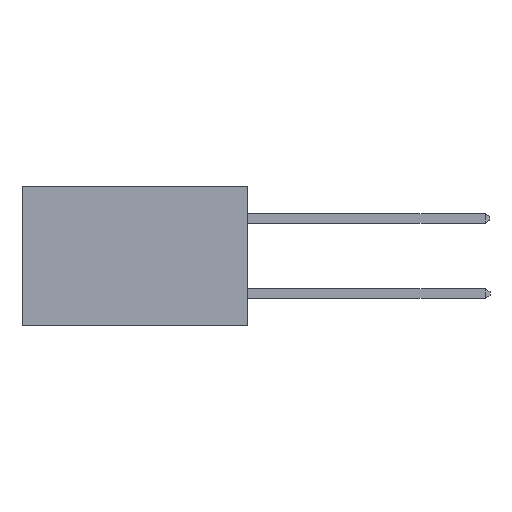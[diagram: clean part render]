
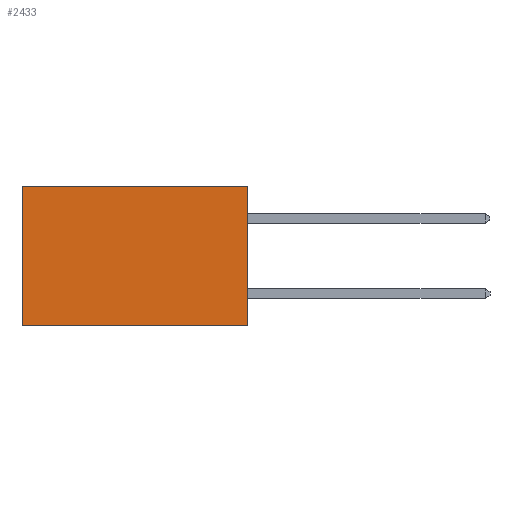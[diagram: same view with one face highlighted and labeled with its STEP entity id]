
A CAD part, left-side view. The second image highlights one B-rep face of the part: STEP entity #2433.
In plain terms, the highlighted planar face has unit normal (-1, 0, 0).
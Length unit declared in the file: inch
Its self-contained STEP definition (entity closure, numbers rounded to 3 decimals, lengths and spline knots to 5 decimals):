
#88 = VECTOR ( 'NONE', #7868, 39.37008 ) ;
#504 = LINE ( 'NONE', #7712, #5541 ) ;
#570 = CARTESIAN_POINT ( 'NONE',  ( 0.2615, 0., 0. ) ) ;
#1166 = CARTESIAN_POINT ( 'NONE',  ( 0.2615, 0.6, -0.37 ) ) ;
#1446 = VECTOR ( 'NONE', #7202, 39.37008 ) ;
#1476 = FACE_OUTER_BOUND ( 'NONE', #3121, .T. ) ;
#1584 = EDGE_CURVE ( 'NONE', #1748, #5989, #6797, .T. ) ;
#1657 = CARTESIAN_POINT ( 'NONE',  ( 0.2615, 0.6, 0. ) ) ;
#1748 = VERTEX_POINT ( 'NONE', #3510 ) ;
#2280 = EDGE_CURVE ( 'NONE', #2652, #6711, #2873, .T. ) ;
#2433 = ADVANCED_FACE ( 'NONE', ( #1476 ), #2938, .F. ) ;
#2652 = VERTEX_POINT ( 'NONE', #570 ) ;
#2756 = AXIS2_PLACEMENT_3D ( 'NONE', #3023, #2908, #2900 ) ;
#2873 = LINE ( 'NONE', #4384, #6101 ) ;
#2900 = DIRECTION ( 'NONE',  ( 0., 0., -1. ) ) ;
#2908 = DIRECTION ( 'NONE',  ( 1., 0., 0. ) ) ;
#2938 = PLANE ( 'NONE',  #2756 ) ;
#3023 = CARTESIAN_POINT ( 'NONE',  ( 0.2615, 0., -0.37 ) ) ;
#3072 = EDGE_CURVE ( 'NONE', #2652, #1748, #504, .T. ) ;
#3121 = EDGE_LOOP ( 'NONE', ( #5852, #5853, #5247, #5927 ) ) ;
#3359 = LINE ( 'NONE', #7219, #1446 ) ;
#3510 = CARTESIAN_POINT ( 'NONE',  ( 0.2615, 0., -0.37 ) ) ;
#3879 = EDGE_CURVE ( 'NONE', #6711, #5989, #3359, .T. ) ;
#4375 = DIRECTION ( 'NONE',  ( 0., 1., 0. ) ) ;
#4384 = CARTESIAN_POINT ( 'NONE',  ( 0.2615, 0., 0. ) ) ;
#5247 = ORIENTED_EDGE ( 'NONE', *, *, #3072, .F. ) ;
#5541 = VECTOR ( 'NONE', #7540, 39.37008 ) ;
#5852 = ORIENTED_EDGE ( 'NONE', *, *, #3879, .T. ) ;
#5853 = ORIENTED_EDGE ( 'NONE', *, *, #1584, .F. ) ;
#5927 = ORIENTED_EDGE ( 'NONE', *, *, #2280, .T. ) ;
#5989 = VERTEX_POINT ( 'NONE', #1166 ) ;
#6101 = VECTOR ( 'NONE', #4375, 39.37008 ) ;
#6711 = VERTEX_POINT ( 'NONE', #1657 ) ;
#6797 = LINE ( 'NONE', #7951, #88 ) ;
#7202 = DIRECTION ( 'NONE',  ( 0., 0., -1. ) ) ;
#7219 = CARTESIAN_POINT ( 'NONE',  ( 0.2615, 0.6, -0.37 ) ) ;
#7540 = DIRECTION ( 'NONE',  ( 0., 0., -1. ) ) ;
#7712 = CARTESIAN_POINT ( 'NONE',  ( 0.2615, 0., -0.37 ) ) ;
#7868 = DIRECTION ( 'NONE',  ( 0., 1., 0. ) ) ;
#7951 = CARTESIAN_POINT ( 'NONE',  ( 0.2615, 0., -0.37 ) ) ;
